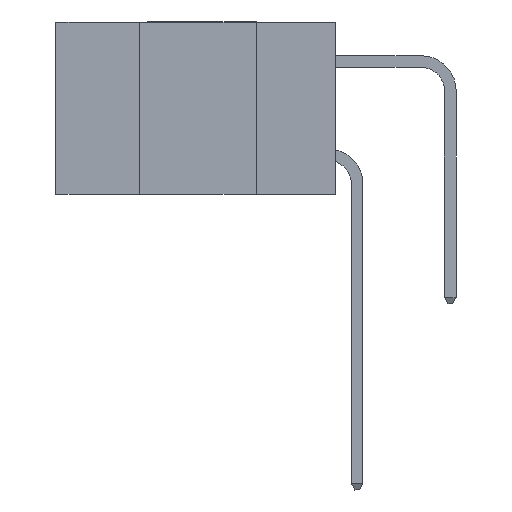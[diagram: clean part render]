
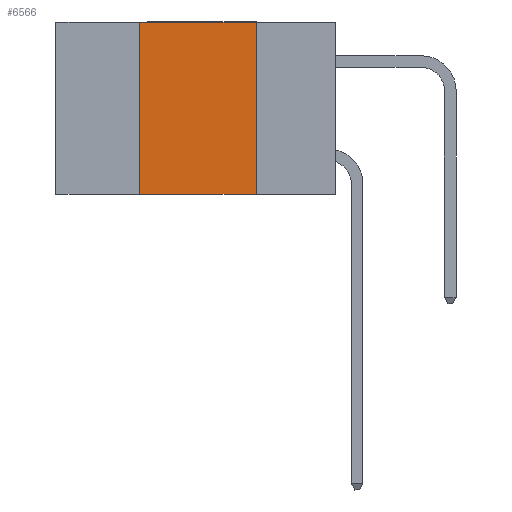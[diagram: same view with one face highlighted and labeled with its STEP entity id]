
A CAD part, left-side view. The second image highlights one B-rep face of the part: STEP entity #6566.
In plain terms, the highlighted planar face has unit normal (-1, 0, 0).
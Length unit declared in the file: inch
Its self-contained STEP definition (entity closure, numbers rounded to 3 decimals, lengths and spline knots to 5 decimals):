
#211 = LINE ( 'NONE', #380, #10667 ) ;
#380 = CARTESIAN_POINT ( 'NONE',  ( 0., 0.6, 0. ) ) ;
#1734 = VERTEX_POINT ( 'NONE', #6270 ) ;
#1882 = ORIENTED_EDGE ( 'NONE', *, *, #9914, .F. ) ;
#1916 = CARTESIAN_POINT ( 'NONE',  ( 0., 0.17, 0. ) ) ;
#1972 = DIRECTION ( 'NONE',  ( 0., 0., -1. ) ) ;
#1980 = VECTOR ( 'NONE', #5038, 39.37008 ) ;
#2144 = VECTOR ( 'NONE', #8616, 39.37008 ) ;
#2380 = EDGE_LOOP ( 'NONE', ( #10501, #1882, #8461, #4417 ) ) ;
#2530 = CARTESIAN_POINT ( 'NONE',  ( 0., 0.6, -0.37 ) ) ;
#2747 = CARTESIAN_POINT ( 'NONE',  ( 0., 0.17, -0.37 ) ) ;
#2773 = VERTEX_POINT ( 'NONE', #3780 ) ;
#3558 = EDGE_CURVE ( 'NONE', #2773, #1734, #6847, .T. ) ;
#3780 = CARTESIAN_POINT ( 'NONE',  ( 0., 0.42, -0.37 ) ) ;
#4221 = EDGE_CURVE ( 'NONE', #2773, #9659, #4264, .T. ) ;
#4264 = LINE ( 'NONE', #2530, #1980 ) ;
#4417 = ORIENTED_EDGE ( 'NONE', *, *, #4221, .T. ) ;
#5038 = DIRECTION ( 'NONE',  ( 0., -1., 0. ) ) ;
#5545 = DIRECTION ( 'NONE',  ( 0., -1., 0. ) ) ;
#5556 = EDGE_CURVE ( 'NONE', #5596, #9659, #10571, .T. ) ;
#5596 = VERTEX_POINT ( 'NONE', #6688 ) ;
#5739 = AXIS2_PLACEMENT_3D ( 'NONE', #9885, #10263, #10236 ) ;
#6270 = CARTESIAN_POINT ( 'NONE',  ( 0., 0.42, 0. ) ) ;
#6566 = ADVANCED_FACE ( 'NONE', ( #9705 ), #10277, .F. ) ;
#6688 = CARTESIAN_POINT ( 'NONE',  ( 0., 0.17, 0. ) ) ;
#6847 = LINE ( 'NONE', #10590, #2144 ) ;
#8461 = ORIENTED_EDGE ( 'NONE', *, *, #3558, .F. ) ;
#8616 = DIRECTION ( 'NONE',  ( 0., 0., 1. ) ) ;
#9007 = VECTOR ( 'NONE', #1972, 39.37008 ) ;
#9659 = VERTEX_POINT ( 'NONE', #2747 ) ;
#9705 = FACE_OUTER_BOUND ( 'NONE', #2380, .T. ) ;
#9885 = CARTESIAN_POINT ( 'NONE',  ( 0., 0.6, 0. ) ) ;
#9914 = EDGE_CURVE ( 'NONE', #1734, #5596, #211, .T. ) ;
#10236 = DIRECTION ( 'NONE',  ( 0., 0., -1. ) ) ;
#10263 = DIRECTION ( 'NONE',  ( 1., 0., 0. ) ) ;
#10277 = PLANE ( 'NONE',  #5739 ) ;
#10501 = ORIENTED_EDGE ( 'NONE', *, *, #5556, .F. ) ;
#10571 = LINE ( 'NONE', #1916, #9007 ) ;
#10590 = CARTESIAN_POINT ( 'NONE',  ( 0., 0.42, 0. ) ) ;
#10667 = VECTOR ( 'NONE', #5545, 39.37008 ) ;
